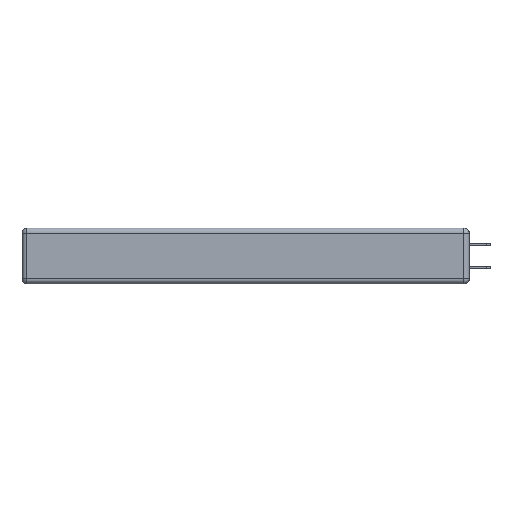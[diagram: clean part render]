
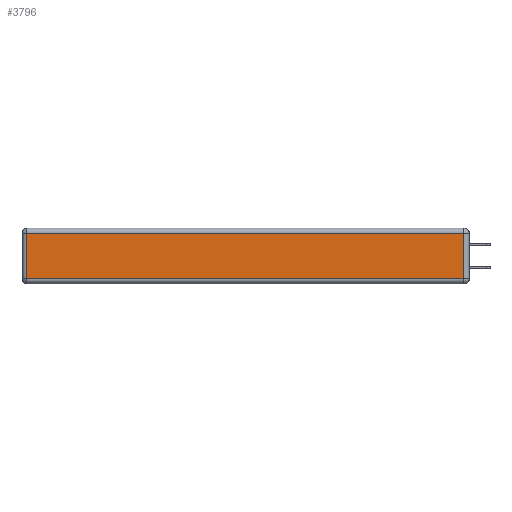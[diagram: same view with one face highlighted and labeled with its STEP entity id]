
A CAD part, left-side view. The second image highlights one B-rep face of the part: STEP entity #3796.
In plain terms, the highlighted planar face has unit normal (-1, 0, 0).
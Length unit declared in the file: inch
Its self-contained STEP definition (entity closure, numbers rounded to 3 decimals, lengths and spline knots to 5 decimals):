
#105 = VECTOR ( 'NONE', #11893, 39.37008 ) ;
#2372 = ORIENTED_EDGE ( 'NONE', *, *, #4514, .T. ) ;
#2941 = LINE ( 'NONE', #5955, #14440 ) ;
#3013 = CARTESIAN_POINT ( 'NONE',  ( 0., 0., -0.313 ) ) ;
#3016 = EDGE_CURVE ( 'NONE', #15685, #9587, #13858, .T. ) ;
#3073 = ORIENTED_EDGE ( 'NONE', *, *, #3016, .T. ) ;
#3281 = CARTESIAN_POINT ( 'NONE',  ( 0., 0., -0.343 ) ) ;
#3332 = VECTOR ( 'NONE', #13703, 39.37008 ) ;
#3592 = ORIENTED_EDGE ( 'NONE', *, *, #6330, .T. ) ;
#3796 = ADVANCED_FACE ( 'NONE', ( #4498 ), #15866, .T. ) ;
#4440 = DIRECTION ( 'NONE',  ( 0., 1., 0. ) ) ;
#4498 = FACE_OUTER_BOUND ( 'NONE', #13354, .T. ) ;
#4514 = EDGE_CURVE ( 'NONE', #9587, #12282, #15587, .T. ) ;
#4564 = DIRECTION ( 'NONE',  ( -1., 0., 0. ) ) ;
#5955 = CARTESIAN_POINT ( 'NONE',  ( 0., 0.03, -0.343 ) ) ;
#6153 = ORIENTED_EDGE ( 'NONE', *, *, #9553, .T. ) ;
#6330 = EDGE_CURVE ( 'NONE', #10349, #15685, #15725, .T. ) ;
#9553 = EDGE_CURVE ( 'NONE', #12282, #10349, #2941, .T. ) ;
#9587 = VERTEX_POINT ( 'NONE', #11147 ) ;
#10270 = CARTESIAN_POINT ( 'NONE',  ( 0., 2.72, -0.343 ) ) ;
#10349 = VERTEX_POINT ( 'NONE', #13362 ) ;
#11019 = CARTESIAN_POINT ( 'NONE',  ( 0., 2.75, -0.03 ) ) ;
#11147 = CARTESIAN_POINT ( 'NONE',  ( 0., 2.72, -0.313 ) ) ;
#11181 = CARTESIAN_POINT ( 'NONE',  ( 0., 2.72, -0.03 ) ) ;
#11893 = DIRECTION ( 'NONE',  ( 0., -1., 0. ) ) ;
#11970 = VECTOR ( 'NONE', #4440, 39.37008 ) ;
#12282 = VERTEX_POINT ( 'NONE', #15974 ) ;
#12569 = DIRECTION ( 'NONE',  ( 0., 0., 1. ) ) ;
#13354 = EDGE_LOOP ( 'NONE', ( #2372, #6153, #3592, #3073 ) ) ;
#13362 = CARTESIAN_POINT ( 'NONE',  ( 0., 0.03, -0.03 ) ) ;
#13703 = DIRECTION ( 'NONE',  ( 0., 0., -1. ) ) ;
#13858 = LINE ( 'NONE', #10270, #3332 ) ;
#14440 = VECTOR ( 'NONE', #12569, 39.37008 ) ;
#14590 = DIRECTION ( 'NONE',  ( 0., 0., 1. ) ) ;
#15587 = LINE ( 'NONE', #3013, #105 ) ;
#15685 = VERTEX_POINT ( 'NONE', #11181 ) ;
#15725 = LINE ( 'NONE', #11019, #11970 ) ;
#15828 = AXIS2_PLACEMENT_3D ( 'NONE', #3281, #4564, #14590 ) ;
#15866 = PLANE ( 'NONE',  #15828 ) ;
#15974 = CARTESIAN_POINT ( 'NONE',  ( 0., 0.03, -0.313 ) ) ;
